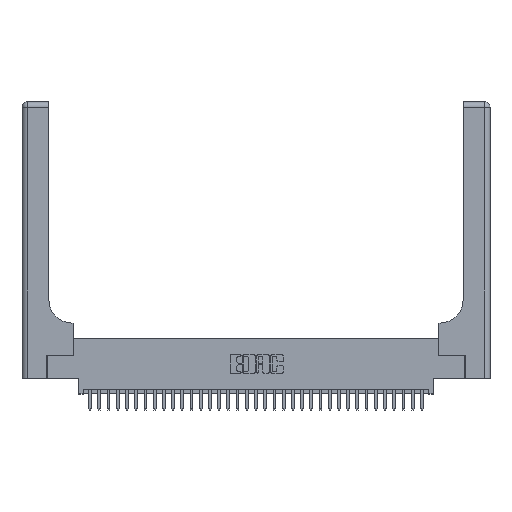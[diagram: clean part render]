
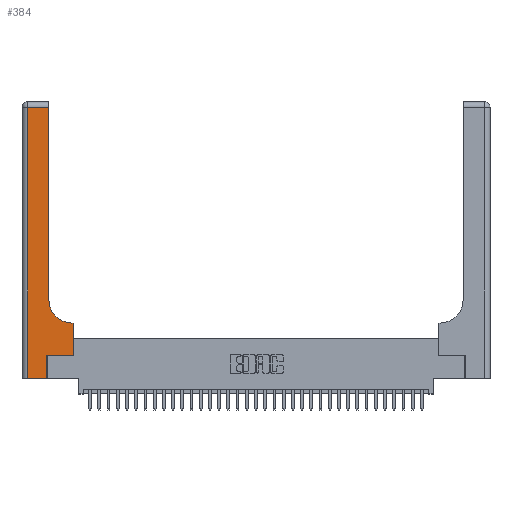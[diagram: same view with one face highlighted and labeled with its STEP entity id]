
A CAD part, top view. The second image highlights one B-rep face of the part: STEP entity #384.
In plain terms, the highlighted planar face has unit normal (0, 0, 1).
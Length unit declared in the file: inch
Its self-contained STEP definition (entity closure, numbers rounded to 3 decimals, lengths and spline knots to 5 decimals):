
#91 = EDGE_CURVE ( 'NONE', #8627, #15105, #13276, .T. ) ;
#384 = ADVANCED_FACE ( 'NONE', ( #32036 ), #23756, .F. ) ;
#1976 = LINE ( 'NONE', #5347, #21955 ) ;
#2560 = DIRECTION ( 'NONE',  ( -1., 0., 0. ) ) ;
#2977 = VERTEX_POINT ( 'NONE', #5875 ) ;
#4400 = LINE ( 'NONE', #12098, #13295 ) ;
#4813 = VECTOR ( 'NONE', #25668, 39.37008 ) ;
#4817 = DIRECTION ( 'NONE',  ( -1., 0., 0. ) ) ;
#4961 = CARTESIAN_POINT ( 'NONE',  ( 0.06, 3., 0.37 ) ) ;
#5168 = ORIENTED_EDGE ( 'NONE', *, *, #26643, .T. ) ;
#5181 = CARTESIAN_POINT ( 'NONE',  ( 0.269, 0.25, 0.37 ) ) ;
#5347 = CARTESIAN_POINT ( 'NONE',  ( 0.2915, 0.6, 0.37 ) ) ;
#5875 = CARTESIAN_POINT ( 'NONE',  ( 0.2915, 2.94, 0.37 ) ) ;
#7526 = EDGE_LOOP ( 'NONE', ( #32636, #19779, #16101, #5168, #30604, #33472, #28945, #30375, #21004 ) ) ;
#7577 = CARTESIAN_POINT ( 'NONE',  ( 0.5585, 0.6, 0.37 ) ) ;
#8041 = DIRECTION ( 'NONE',  ( 1., 0., 0. ) ) ;
#8070 = CARTESIAN_POINT ( 'NONE',  ( 0.5415, 0.6, 0.37 ) ) ;
#8414 = AXIS2_PLACEMENT_3D ( 'NONE', #26356, #10295, #4817 ) ;
#8432 = LINE ( 'NONE', #5181, #27999 ) ;
#8578 = EDGE_CURVE ( 'NONE', #30329, #19397, #4400, .T. ) ;
#8627 = VERTEX_POINT ( 'NONE', #19356 ) ;
#10295 = DIRECTION ( 'NONE',  ( 0., 0., -1. ) ) ;
#11361 = VERTEX_POINT ( 'NONE', #8070 ) ;
#12098 = CARTESIAN_POINT ( 'NONE',  ( 0.5585, 0.25, 0.37 ) ) ;
#12165 = DIRECTION ( 'NONE',  ( 1., 0., 0. ) ) ;
#12405 = CARTESIAN_POINT ( 'NONE',  ( 0.2915, 0.85, 0.37 ) ) ;
#13021 = DIRECTION ( 'NONE',  ( 0., -1., 0. ) ) ;
#13276 = LINE ( 'NONE', #20466, #4813 ) ;
#13295 = VECTOR ( 'NONE', #27235, 39.37008 ) ;
#13315 = VERTEX_POINT ( 'NONE', #24987 ) ;
#14339 = VECTOR ( 'NONE', #2560, 39.37008 ) ;
#15009 = EDGE_CURVE ( 'NONE', #2977, #19255, #25462, .T. ) ;
#15105 = VERTEX_POINT ( 'NONE', #29346 ) ;
#16000 = VECTOR ( 'NONE', #29804, 39.37008 ) ;
#16101 = ORIENTED_EDGE ( 'NONE', *, *, #33185, .T. ) ;
#18695 = DIRECTION ( 'NONE',  ( -1., 0., 0. ) ) ;
#18806 = LINE ( 'NONE', #29701, #33624 ) ;
#18829 = CARTESIAN_POINT ( 'NONE',  ( 0.2915, 3., 0.37 ) ) ;
#18936 = AXIS2_PLACEMENT_3D ( 'NONE', #28503, #23272, #12165 ) ;
#19255 = VERTEX_POINT ( 'NONE', #23287 ) ;
#19356 = CARTESIAN_POINT ( 'NONE',  ( 0.269, 0., 0.37 ) ) ;
#19397 = VERTEX_POINT ( 'NONE', #7577 ) ;
#19751 = LINE ( 'NONE', #18829, #16000 ) ;
#19779 = ORIENTED_EDGE ( 'NONE', *, *, #15009, .T. ) ;
#20466 = CARTESIAN_POINT ( 'NONE',  ( 0.269, 0., 0.37 ) ) ;
#21004 = ORIENTED_EDGE ( 'NONE', *, *, #24443, .T. ) ;
#21788 = LINE ( 'NONE', #4961, #22645 ) ;
#21955 = VECTOR ( 'NONE', #18695, 39.37008 ) ;
#22101 = EDGE_CURVE ( 'NONE', #15105, #30329, #8432, .T. ) ;
#22645 = VECTOR ( 'NONE', #13021, 39.37008 ) ;
#23272 = DIRECTION ( 'NONE',  ( 0., 0., -1. ) ) ;
#23287 = CARTESIAN_POINT ( 'NONE',  ( 0.06, 2.94, 0.37 ) ) ;
#23756 = PLANE ( 'NONE',  #8414 ) ;
#24099 = CIRCLE ( 'NONE', #18936, 0.25 ) ;
#24204 = CARTESIAN_POINT ( 'NONE',  ( 0., 2.94, 0.37 ) ) ;
#24309 = VERTEX_POINT ( 'NONE', #12405 ) ;
#24443 = EDGE_CURVE ( 'NONE', #11361, #24309, #24099, .T. ) ;
#24715 = EDGE_CURVE ( 'NONE', #24309, #2977, #19751, .T. ) ;
#24987 = CARTESIAN_POINT ( 'NONE',  ( 0.06, 0., 0.37 ) ) ;
#25462 = LINE ( 'NONE', #24204, #14339 ) ;
#25668 = DIRECTION ( 'NONE',  ( 0., 1., 0. ) ) ;
#26356 = CARTESIAN_POINT ( 'NONE',  ( 0., 3., 0.37 ) ) ;
#26643 = EDGE_CURVE ( 'NONE', #13315, #8627, #18806, .T. ) ;
#27037 = DIRECTION ( 'NONE',  ( 1., 0., 0. ) ) ;
#27235 = DIRECTION ( 'NONE',  ( 0., 1., 0. ) ) ;
#27999 = VECTOR ( 'NONE', #8041, 39.37008 ) ;
#28503 = CARTESIAN_POINT ( 'NONE',  ( 0.5415, 0.85, 0.37 ) ) ;
#28945 = ORIENTED_EDGE ( 'NONE', *, *, #8578, .T. ) ;
#29346 = CARTESIAN_POINT ( 'NONE',  ( 0.269, 0.25, 0.37 ) ) ;
#29701 = CARTESIAN_POINT ( 'NONE',  ( 0., 0., 0.37 ) ) ;
#29804 = DIRECTION ( 'NONE',  ( 0., 1., 0. ) ) ;
#30329 = VERTEX_POINT ( 'NONE', #34542 ) ;
#30375 = ORIENTED_EDGE ( 'NONE', *, *, #31601, .T. ) ;
#30604 = ORIENTED_EDGE ( 'NONE', *, *, #91, .T. ) ;
#31601 = EDGE_CURVE ( 'NONE', #19397, #11361, #1976, .T. ) ;
#32036 = FACE_OUTER_BOUND ( 'NONE', #7526, .T. ) ;
#32636 = ORIENTED_EDGE ( 'NONE', *, *, #24715, .T. ) ;
#33185 = EDGE_CURVE ( 'NONE', #19255, #13315, #21788, .T. ) ;
#33472 = ORIENTED_EDGE ( 'NONE', *, *, #22101, .T. ) ;
#33624 = VECTOR ( 'NONE', #27037, 39.37008 ) ;
#34542 = CARTESIAN_POINT ( 'NONE',  ( 0.5585, 0.25, 0.37 ) ) ;
